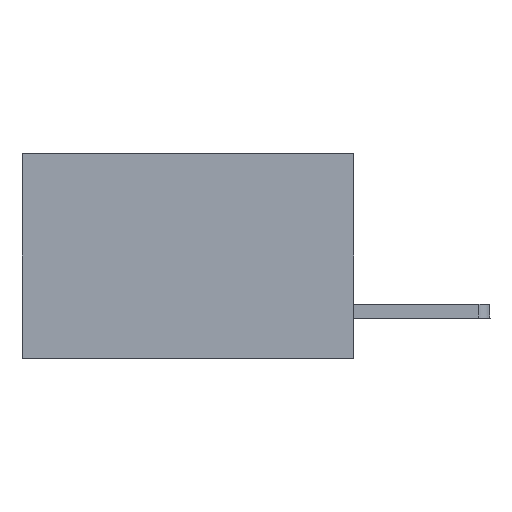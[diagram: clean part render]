
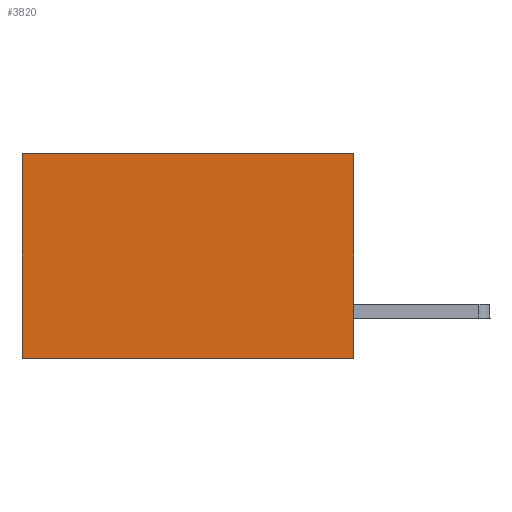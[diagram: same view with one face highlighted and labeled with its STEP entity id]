
A CAD part, left-side view. The second image highlights one B-rep face of the part: STEP entity #3820.
In plain terms, the highlighted planar face has unit normal (-1, 0, 0).
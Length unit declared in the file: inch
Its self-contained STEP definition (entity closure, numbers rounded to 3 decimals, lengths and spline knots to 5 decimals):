
#21 = VERTEX_POINT ( 'NONE', #2016 ) ;
#212 = CARTESIAN_POINT ( 'NONE',  ( 0.2875, 0., 0. ) ) ;
#392 = VECTOR ( 'NONE', #13499, 39.37008 ) ;
#862 = DIRECTION ( 'NONE',  ( 0., 0., -1. ) ) ;
#1247 = ORIENTED_EDGE ( 'NONE', *, *, #9627, .F. ) ;
#1683 = PLANE ( 'NONE',  #9216 ) ;
#1930 = LINE ( 'NONE', #6704, #7623 ) ;
#1941 = EDGE_LOOP ( 'NONE', ( #9095, #9417, #1247, #7366 ) ) ;
#2016 = CARTESIAN_POINT ( 'NONE',  ( 0.2875, 0.6, 0. ) ) ;
#2734 = CARTESIAN_POINT ( 'NONE',  ( 0.2875, 0., 0. ) ) ;
#2767 = EDGE_CURVE ( 'NONE', #21, #5463, #6713, .T. ) ;
#3820 = ADVANCED_FACE ( 'NONE', ( #4045 ), #1683, .F. ) ;
#3985 = LINE ( 'NONE', #4343, #392 ) ;
#4045 = FACE_OUTER_BOUND ( 'NONE', #1941, .T. ) ;
#4229 = DIRECTION ( 'NONE',  ( 0., 1., 0. ) ) ;
#4343 = CARTESIAN_POINT ( 'NONE',  ( 0.2875, 0., -0.37 ) ) ;
#5463 = VERTEX_POINT ( 'NONE', #12799 ) ;
#5502 = DIRECTION ( 'NONE',  ( 0., 0., -1. ) ) ;
#5529 = CARTESIAN_POINT ( 'NONE',  ( 0.2875, 0.6, 0. ) ) ;
#5646 = EDGE_CURVE ( 'NONE', #9121, #5463, #3985, .T. ) ;
#6323 = DIRECTION ( 'NONE',  ( 0., 0., -1. ) ) ;
#6379 = VECTOR ( 'NONE', #4229, 39.37008 ) ;
#6704 = CARTESIAN_POINT ( 'NONE',  ( 0.2875, 0., 0. ) ) ;
#6713 = LINE ( 'NONE', #5529, #9398 ) ;
#7366 = ORIENTED_EDGE ( 'NONE', *, *, #8695, .T. ) ;
#7623 = VECTOR ( 'NONE', #862, 39.37008 ) ;
#8526 = CARTESIAN_POINT ( 'NONE',  ( 0.2875, 0., 0. ) ) ;
#8695 = EDGE_CURVE ( 'NONE', #11460, #21, #9704, .T. ) ;
#9051 = CARTESIAN_POINT ( 'NONE',  ( 0.2875, 0., -0.37 ) ) ;
#9095 = ORIENTED_EDGE ( 'NONE', *, *, #2767, .T. ) ;
#9121 = VERTEX_POINT ( 'NONE', #9051 ) ;
#9216 = AXIS2_PLACEMENT_3D ( 'NONE', #2734, #12255, #6323 ) ;
#9398 = VECTOR ( 'NONE', #5502, 39.37008 ) ;
#9417 = ORIENTED_EDGE ( 'NONE', *, *, #5646, .F. ) ;
#9627 = EDGE_CURVE ( 'NONE', #11460, #9121, #1930, .T. ) ;
#9704 = LINE ( 'NONE', #8526, #6379 ) ;
#11460 = VERTEX_POINT ( 'NONE', #212 ) ;
#12255 = DIRECTION ( 'NONE',  ( 1., 0., 0. ) ) ;
#12799 = CARTESIAN_POINT ( 'NONE',  ( 0.2875, 0.6, -0.37 ) ) ;
#13499 = DIRECTION ( 'NONE',  ( 0., 1., 0. ) ) ;
